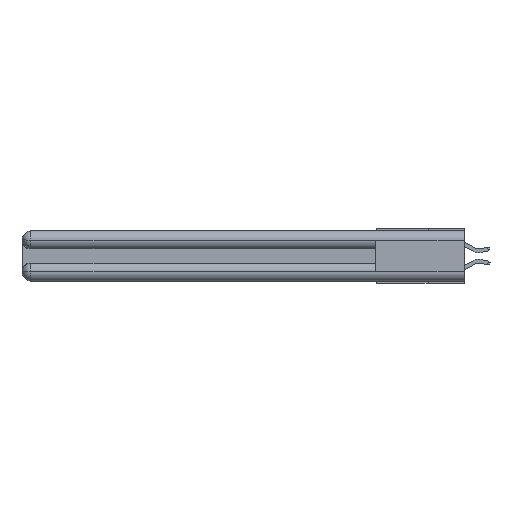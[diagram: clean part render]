
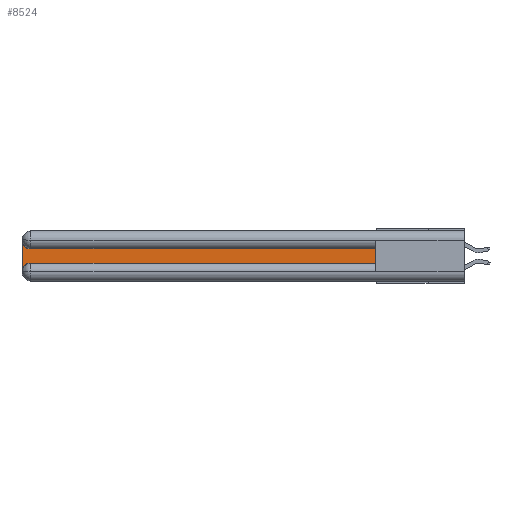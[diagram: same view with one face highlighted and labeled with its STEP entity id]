
A CAD part, left-side view. The second image highlights one B-rep face of the part: STEP entity #8524.
In plain terms, the highlighted planar face has unit normal (-1, 0, 0).
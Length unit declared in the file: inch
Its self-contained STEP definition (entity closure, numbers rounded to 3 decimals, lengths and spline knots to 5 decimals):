
#391 = DIRECTION ( 'NONE',  ( 0., 0., -1. ) ) ;
#582 = DIRECTION ( 'NONE',  ( 0., 0., 1. ) ) ;
#821 = VERTEX_POINT ( 'NONE', #29945 ) ;
#2773 = EDGE_CURVE ( 'NONE', #821, #13943, #31513, .T. ) ;
#2956 = AXIS2_PLACEMENT_3D ( 'NONE', #23540, #34576, #29097 ) ;
#3154 = ORIENTED_EDGE ( 'NONE', *, *, #9010, .T. ) ;
#4269 = EDGE_CURVE ( 'NONE', #28311, #31493, #6102, .T. ) ;
#4357 = VERTEX_POINT ( 'NONE', #29329 ) ;
#5210 = EDGE_CURVE ( 'NONE', #13943, #28311, #33069, .T. ) ;
#5583 = CARTESIAN_POINT ( 'NONE',  ( 0.075, 2.94, -0.2775 ) ) ;
#6102 = CIRCLE ( 'NONE', #10330, 0.06 ) ;
#6532 = VECTOR ( 'NONE', #9656, 39.37008 ) ;
#6799 = ORIENTED_EDGE ( 'NONE', *, *, #26548, .T. ) ;
#8524 = ADVANCED_FACE ( 'NONE', ( #21886 ), #10077, .F. ) ;
#8529 = LINE ( 'NONE', #16785, #10270 ) ;
#9010 = EDGE_CURVE ( 'NONE', #4357, #22196, #9871, .T. ) ;
#9656 = DIRECTION ( 'NONE',  ( 0., 1., 0. ) ) ;
#9729 = DIRECTION ( 'NONE',  ( 1., 0., 0. ) ) ;
#9871 = CIRCLE ( 'NONE', #29322, 0.06 ) ;
#10077 = PLANE ( 'NONE',  #2956 ) ;
#10270 = VECTOR ( 'NONE', #391, 39.37008 ) ;
#10330 = AXIS2_PLACEMENT_3D ( 'NONE', #14929, #9729, #28865 ) ;
#12023 = ORIENTED_EDGE ( 'NONE', *, *, #5210, .T. ) ;
#12677 = CARTESIAN_POINT ( 'NONE',  ( 0.075, 2.94, -0.2175 ) ) ;
#13943 = VERTEX_POINT ( 'NONE', #23632 ) ;
#14513 = ORIENTED_EDGE ( 'NONE', *, *, #2773, .T. ) ;
#14929 = CARTESIAN_POINT ( 'NONE',  ( 0.075, 2.94, -0.0625 ) ) ;
#15941 = CARTESIAN_POINT ( 'NONE',  ( 0.075, 3., -0.0625 ) ) ;
#16785 = CARTESIAN_POINT ( 'NONE',  ( 0.075, 3., -0.2175 ) ) ;
#17481 = EDGE_CURVE ( 'NONE', #31493, #4357, #8529, .T. ) ;
#17655 = LINE ( 'NONE', #33537, #34793 ) ;
#17848 = CARTESIAN_POINT ( 'NONE',  ( 0.075, 0.6, -0.1225 ) ) ;
#19474 = EDGE_LOOP ( 'NONE', ( #12023, #35026, #26951, #3154, #6799, #14513 ) ) ;
#20219 = DIRECTION ( 'NONE',  ( 0., -1., 0. ) ) ;
#21886 = FACE_OUTER_BOUND ( 'NONE', #19474, .T. ) ;
#22196 = VERTEX_POINT ( 'NONE', #12677 ) ;
#23540 = CARTESIAN_POINT ( 'NONE',  ( 0.075, 3., -0.1225 ) ) ;
#23632 = CARTESIAN_POINT ( 'NONE',  ( 0.075, 0.6, -0.1225 ) ) ;
#24471 = CARTESIAN_POINT ( 'NONE',  ( 0.075, 2.94, -0.1225 ) ) ;
#26548 = EDGE_CURVE ( 'NONE', #22196, #821, #17655, .T. ) ;
#26951 = ORIENTED_EDGE ( 'NONE', *, *, #17481, .T. ) ;
#27890 = CARTESIAN_POINT ( 'NONE',  ( 0.075, 0.6, -0.2175 ) ) ;
#28311 = VERTEX_POINT ( 'NONE', #24471 ) ;
#28865 = DIRECTION ( 'NONE',  ( 0., 0., -1. ) ) ;
#29097 = DIRECTION ( 'NONE',  ( 0., 0., -1. ) ) ;
#29322 = AXIS2_PLACEMENT_3D ( 'NONE', #5583, #32876, #35235 ) ;
#29329 = CARTESIAN_POINT ( 'NONE',  ( 0.075, 3., -0.2775 ) ) ;
#29945 = CARTESIAN_POINT ( 'NONE',  ( 0.075, 0.6, -0.2175 ) ) ;
#30662 = VECTOR ( 'NONE', #582, 39.37008 ) ;
#31493 = VERTEX_POINT ( 'NONE', #15941 ) ;
#31513 = LINE ( 'NONE', #27890, #30662 ) ;
#32876 = DIRECTION ( 'NONE',  ( 1., 0., 0. ) ) ;
#33069 = LINE ( 'NONE', #17848, #6532 ) ;
#33537 = CARTESIAN_POINT ( 'NONE',  ( 0.075, 0.6, -0.2175 ) ) ;
#34576 = DIRECTION ( 'NONE',  ( 1., 0., 0. ) ) ;
#34793 = VECTOR ( 'NONE', #20219, 39.37008 ) ;
#35026 = ORIENTED_EDGE ( 'NONE', *, *, #4269, .T. ) ;
#35235 = DIRECTION ( 'NONE',  ( 0., 0., -1. ) ) ;
